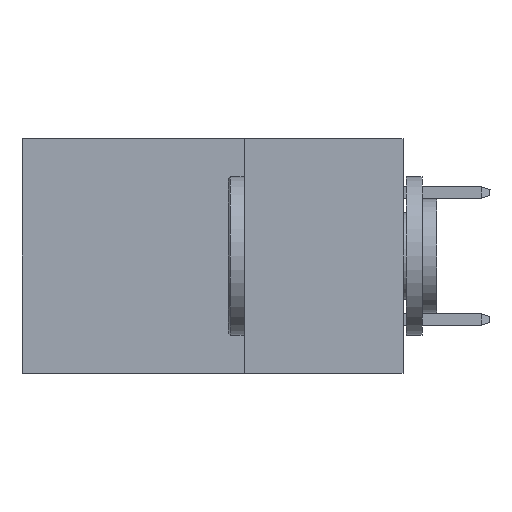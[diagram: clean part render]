
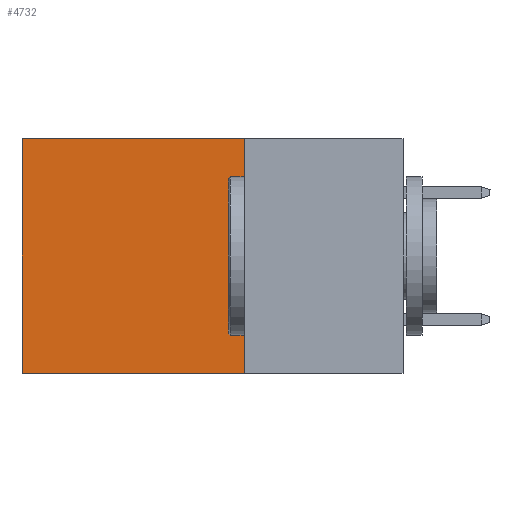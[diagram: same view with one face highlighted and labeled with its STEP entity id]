
A CAD part, left-side view. The second image highlights one B-rep face of the part: STEP entity #4732.
In plain terms, the highlighted planar face has unit normal (-1, 0, 0).
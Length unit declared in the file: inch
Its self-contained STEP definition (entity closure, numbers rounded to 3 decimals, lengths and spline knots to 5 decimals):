
#3969 = EDGE_CURVE ( 'NONE', #29723, #18339, #28702, .T. ) ;
#4732 = ADVANCED_FACE ( 'NONE', ( #30946 ), #42089, .F. ) ;
#6508 = ORIENTED_EDGE ( 'NONE', *, *, #7305, .F. ) ;
#7305 = EDGE_CURVE ( 'NONE', #35724, #18339, #36951, .T. ) ;
#7901 = CARTESIAN_POINT ( 'NONE',  ( 0.2875, 0.6, -0.37 ) ) ;
#9758 = CARTESIAN_POINT ( 'NONE',  ( 0.2875, 0.25, 0. ) ) ;
#9794 = DIRECTION ( 'NONE',  ( 0., 1., 0. ) ) ;
#10227 = DIRECTION ( 'NONE',  ( 0., 0., -1. ) ) ;
#15141 = DIRECTION ( 'NONE',  ( 0., 0., -1. ) ) ;
#15710 = ORIENTED_EDGE ( 'NONE', *, *, #23199, .F. ) ;
#16158 = CARTESIAN_POINT ( 'NONE',  ( 0.2875, 0.25, -0.37 ) ) ;
#17941 = LINE ( 'NONE', #31508, #34038 ) ;
#18339 = VERTEX_POINT ( 'NONE', #7901 ) ;
#20445 = CARTESIAN_POINT ( 'NONE',  ( 0.2875, 0.25, 0. ) ) ;
#21427 = LINE ( 'NONE', #9758, #40521 ) ;
#21858 = EDGE_LOOP ( 'NONE', ( #35967, #6508, #15710, #35505 ) ) ;
#23199 = EDGE_CURVE ( 'NONE', #42276, #35724, #21427, .T. ) ;
#23790 = CARTESIAN_POINT ( 'NONE',  ( 0.2875, 0.25, -0.37 ) ) ;
#25188 = AXIS2_PLACEMENT_3D ( 'NONE', #20445, #41620, #31395 ) ;
#25364 = CARTESIAN_POINT ( 'NONE',  ( 0.2875, 0.6, 0. ) ) ;
#27661 = EDGE_CURVE ( 'NONE', #42276, #29723, #17941, .T. ) ;
#28052 = VECTOR ( 'NONE', #15141, 39.37008 ) ;
#28455 = CARTESIAN_POINT ( 'NONE',  ( 0.2875, 0.6, 0. ) ) ;
#28702 = LINE ( 'NONE', #28455, #28052 ) ;
#29723 = VERTEX_POINT ( 'NONE', #25364 ) ;
#30946 = FACE_OUTER_BOUND ( 'NONE', #21858, .T. ) ;
#31395 = DIRECTION ( 'NONE',  ( 0., 0., -1. ) ) ;
#31508 = CARTESIAN_POINT ( 'NONE',  ( 0.2875, 0.25, 0. ) ) ;
#34038 = VECTOR ( 'NONE', #9794, 39.37008 ) ;
#35505 = ORIENTED_EDGE ( 'NONE', *, *, #27661, .T. ) ;
#35724 = VERTEX_POINT ( 'NONE', #23790 ) ;
#35967 = ORIENTED_EDGE ( 'NONE', *, *, #3969, .T. ) ;
#36951 = LINE ( 'NONE', #16158, #43212 ) ;
#40521 = VECTOR ( 'NONE', #10227, 39.37008 ) ;
#41078 = DIRECTION ( 'NONE',  ( 0., 1., 0. ) ) ;
#41620 = DIRECTION ( 'NONE',  ( 1., 0., 0. ) ) ;
#42089 = PLANE ( 'NONE',  #25188 ) ;
#42276 = VERTEX_POINT ( 'NONE', #43252 ) ;
#43212 = VECTOR ( 'NONE', #41078, 39.37008 ) ;
#43252 = CARTESIAN_POINT ( 'NONE',  ( 0.2875, 0.25, 0. ) ) ;
